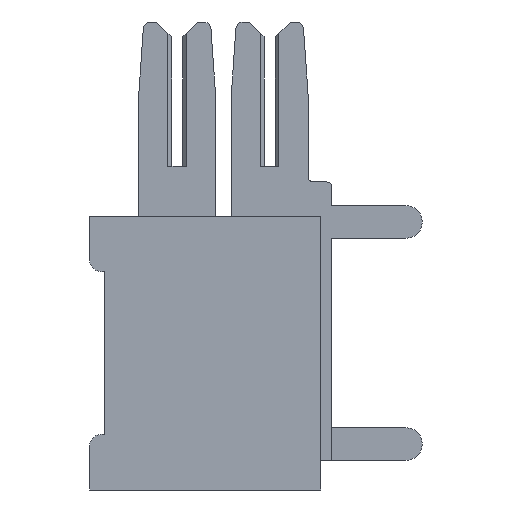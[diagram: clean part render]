
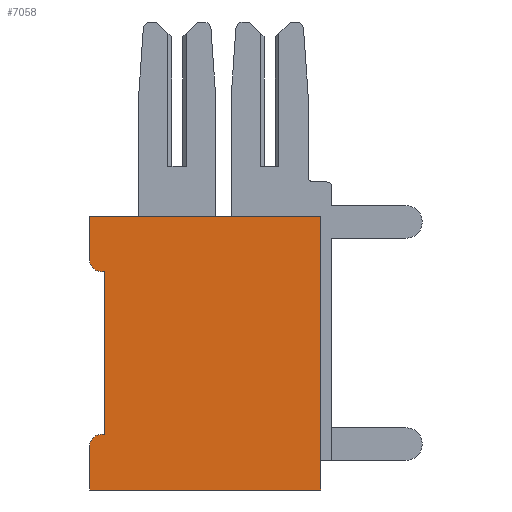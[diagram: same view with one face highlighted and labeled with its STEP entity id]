
A CAD part, left-side view. The second image highlights one B-rep face of the part: STEP entity #7058.
In plain terms, the highlighted planar face has unit normal (-1, 0, 0).
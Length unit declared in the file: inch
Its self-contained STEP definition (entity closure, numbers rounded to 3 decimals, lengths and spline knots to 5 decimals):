
#216 = CARTESIAN_POINT ( 'NONE',  ( 0., 0., -0.37 ) ) ;
#253 = EDGE_CURVE ( 'NONE', #897, #2615, #6038, .T. ) ;
#281 = FACE_OUTER_BOUND ( 'NONE', #4548, .T. ) ;
#439 = DIRECTION ( 'NONE',  ( 0., -1., 0. ) ) ;
#502 = ORIENTED_EDGE ( 'NONE', *, *, #253, .F. ) ;
#661 = VECTOR ( 'NONE', #5213, 39.37008 ) ;
#681 = ORIENTED_EDGE ( 'NONE', *, *, #7162, .F. ) ;
#723 = CARTESIAN_POINT ( 'NONE',  ( 0., 0.312, -0.075 ) ) ;
#897 = VERTEX_POINT ( 'NONE', #6145 ) ;
#923 = LINE ( 'NONE', #2709, #5945 ) ;
#1038 = CARTESIAN_POINT ( 'NONE',  ( 0., 0.292, -0.295 ) ) ;
#1053 = ORIENTED_EDGE ( 'NONE', *, *, #4637, .T. ) ;
#1183 = EDGE_CURVE ( 'NONE', #7809, #1854, #6146, .T. ) ;
#1427 = DIRECTION ( 'NONE',  ( -1., 0., 0. ) ) ;
#1471 = VECTOR ( 'NONE', #2053, 39.37008 ) ;
#1508 = LINE ( 'NONE', #723, #3635 ) ;
#1717 = ORIENTED_EDGE ( 'NONE', *, *, #5191, .T. ) ;
#1727 = CARTESIAN_POINT ( 'NONE',  ( 0., 0.297, -0.31 ) ) ;
#1854 = VERTEX_POINT ( 'NONE', #4153 ) ;
#1907 = EDGE_CURVE ( 'NONE', #6585, #1854, #2176, .T. ) ;
#2014 = AXIS2_PLACEMENT_3D ( 'NONE', #7314, #7289, #4250 ) ;
#2053 = DIRECTION ( 'NONE',  ( 0., -1., 0. ) ) ;
#2056 = LINE ( 'NONE', #7733, #3121 ) ;
#2057 = PLANE ( 'NONE',  #2182 ) ;
#2176 = CIRCLE ( 'NONE', #4590, 0.015 ) ;
#2182 = AXIS2_PLACEMENT_3D ( 'NONE', #216, #1427, #6290 ) ;
#2289 = EDGE_CURVE ( 'NONE', #2615, #4949, #5942, .T. ) ;
#2331 = CARTESIAN_POINT ( 'NONE',  ( 0., 0.312, -0.37 ) ) ;
#2483 = ORIENTED_EDGE ( 'NONE', *, *, #2289, .F. ) ;
#2485 = CARTESIAN_POINT ( 'NONE',  ( 0., 0.312, -0.37 ) ) ;
#2615 = VERTEX_POINT ( 'NONE', #5460 ) ;
#2709 = CARTESIAN_POINT ( 'NONE',  ( 0., 0., -0.37 ) ) ;
#2797 = DIRECTION ( 'NONE',  ( 0., 0., 1. ) ) ;
#2841 = VECTOR ( 'NONE', #6503, 39.37008 ) ;
#3116 = DIRECTION ( 'NONE',  ( 0., 1., 0. ) ) ;
#3121 = VECTOR ( 'NONE', #439, 39.37008 ) ;
#3253 = ORIENTED_EDGE ( 'NONE', *, *, #1907, .T. ) ;
#3348 = CARTESIAN_POINT ( 'NONE',  ( 0., 0.297, -0.075 ) ) ;
#3529 = CARTESIAN_POINT ( 'NONE',  ( 0., 0.312, -0.37 ) ) ;
#3600 = EDGE_CURVE ( 'NONE', #6585, #4379, #2056, .T. ) ;
#3635 = VECTOR ( 'NONE', #3116, 39.37008 ) ;
#3667 = ORIENTED_EDGE ( 'NONE', *, *, #6876, .F. ) ;
#3762 = EDGE_CURVE ( 'NONE', #7809, #5151, #4624, .T. ) ;
#3970 = CARTESIAN_POINT ( 'NONE',  ( 0., 0.292, -0.075 ) ) ;
#4017 = ORIENTED_EDGE ( 'NONE', *, *, #3762, .T. ) ;
#4116 = CARTESIAN_POINT ( 'NONE',  ( 0., 0., 0. ) ) ;
#4153 = CARTESIAN_POINT ( 'NONE',  ( 0., 0.312, -0.31 ) ) ;
#4250 = DIRECTION ( 'NONE',  ( 0., 0., 1. ) ) ;
#4379 = VERTEX_POINT ( 'NONE', #6881 ) ;
#4443 = CIRCLE ( 'NONE', #2014, 0.015 ) ;
#4548 = EDGE_LOOP ( 'NONE', ( #502, #1717, #3667, #681, #6660, #3253, #5679, #4017, #1053, #2483 ) ) ;
#4549 = VECTOR ( 'NONE', #6693, 39.37008 ) ;
#4590 = AXIS2_PLACEMENT_3D ( 'NONE', #1727, #7191, #2797 ) ;
#4624 = LINE ( 'NONE', #5240, #2841 ) ;
#4637 = EDGE_CURVE ( 'NONE', #5151, #4949, #923, .T. ) ;
#4642 = DIRECTION ( 'NONE',  ( 0., 0., 1. ) ) ;
#4760 = DIRECTION ( 'NONE',  ( 0., 0., 1. ) ) ;
#4920 = VERTEX_POINT ( 'NONE', #3348 ) ;
#4949 = VERTEX_POINT ( 'NONE', #4116 ) ;
#5151 = VERTEX_POINT ( 'NONE', #5399 ) ;
#5191 = EDGE_CURVE ( 'NONE', #897, #4920, #4443, .T. ) ;
#5213 = DIRECTION ( 'NONE',  ( 0., 0., 1. ) ) ;
#5240 = CARTESIAN_POINT ( 'NONE',  ( 0., 0., -0.37 ) ) ;
#5399 = CARTESIAN_POINT ( 'NONE',  ( 0., 0., -0.37 ) ) ;
#5460 = CARTESIAN_POINT ( 'NONE',  ( 0., 0.312, 0. ) ) ;
#5671 = CARTESIAN_POINT ( 'NONE',  ( 0., 0., 0. ) ) ;
#5679 = ORIENTED_EDGE ( 'NONE', *, *, #1183, .F. ) ;
#5922 = CARTESIAN_POINT ( 'NONE',  ( 0., 0.297, -0.295 ) ) ;
#5942 = LINE ( 'NONE', #5671, #1471 ) ;
#5945 = VECTOR ( 'NONE', #4642, 39.37008 ) ;
#6038 = LINE ( 'NONE', #3529, #6612 ) ;
#6145 = CARTESIAN_POINT ( 'NONE',  ( 0., 0.312, -0.06 ) ) ;
#6146 = LINE ( 'NONE', #2485, #4549 ) ;
#6290 = DIRECTION ( 'NONE',  ( 0., 0., 1. ) ) ;
#6503 = DIRECTION ( 'NONE',  ( 0., -1., 0. ) ) ;
#6523 = VERTEX_POINT ( 'NONE', #3970 ) ;
#6585 = VERTEX_POINT ( 'NONE', #5922 ) ;
#6612 = VECTOR ( 'NONE', #4760, 39.37008 ) ;
#6660 = ORIENTED_EDGE ( 'NONE', *, *, #3600, .F. ) ;
#6693 = DIRECTION ( 'NONE',  ( 0., 0., 1. ) ) ;
#6876 = EDGE_CURVE ( 'NONE', #6523, #4920, #1508, .T. ) ;
#6881 = CARTESIAN_POINT ( 'NONE',  ( 0., 0.292, -0.295 ) ) ;
#7058 = ADVANCED_FACE ( 'NONE', ( #281 ), #2057, .T. ) ;
#7162 = EDGE_CURVE ( 'NONE', #4379, #6523, #7322, .T. ) ;
#7191 = DIRECTION ( 'NONE',  ( -1., 0., 0. ) ) ;
#7289 = DIRECTION ( 'NONE',  ( -1., 0., 0. ) ) ;
#7314 = CARTESIAN_POINT ( 'NONE',  ( 0., 0.297, -0.06 ) ) ;
#7322 = LINE ( 'NONE', #1038, #661 ) ;
#7733 = CARTESIAN_POINT ( 'NONE',  ( 0., 0.312, -0.295 ) ) ;
#7809 = VERTEX_POINT ( 'NONE', #2331 ) ;
